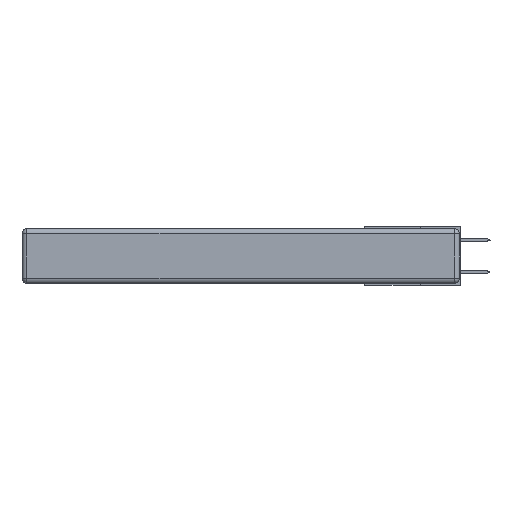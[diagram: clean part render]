
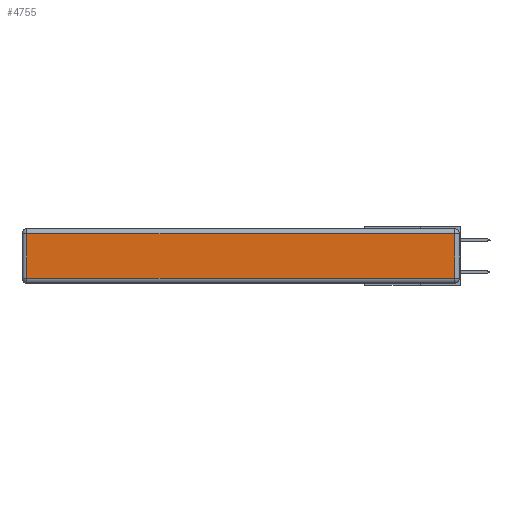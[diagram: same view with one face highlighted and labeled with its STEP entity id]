
A CAD part, left-side view. The second image highlights one B-rep face of the part: STEP entity #4755.
In plain terms, the highlighted planar face has unit normal (-1, 0, 0).
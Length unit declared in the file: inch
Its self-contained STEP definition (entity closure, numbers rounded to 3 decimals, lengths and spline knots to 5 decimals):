
#144 = VECTOR ( 'NONE', #8785, 39.37008 ) ;
#2497 = EDGE_CURVE ( 'NONE', #9733, #4159, #14385, .T. ) ;
#2549 = CARTESIAN_POINT ( 'NONE',  ( 0., 0.03, -0.313 ) ) ;
#3283 = LINE ( 'NONE', #12696, #7405 ) ;
#3413 = VECTOR ( 'NONE', #4306, 39.37008 ) ;
#3564 = DIRECTION ( 'NONE',  ( 0., 1., 0. ) ) ;
#3847 = LINE ( 'NONE', #7568, #144 ) ;
#4159 = VERTEX_POINT ( 'NONE', #8038 ) ;
#4306 = DIRECTION ( 'NONE',  ( 0., -1., 0. ) ) ;
#4515 = ORIENTED_EDGE ( 'NONE', *, *, #11429, .T. ) ;
#4755 = ADVANCED_FACE ( 'NONE', ( #17570 ), #12852, .T. ) ;
#5705 = ORIENTED_EDGE ( 'NONE', *, *, #2497, .T. ) ;
#7132 = CARTESIAN_POINT ( 'NONE',  ( 0., 2.72, -0.313 ) ) ;
#7305 = DIRECTION ( 'NONE',  ( 0., 0., 1. ) ) ;
#7405 = VECTOR ( 'NONE', #14125, 39.37008 ) ;
#7568 = CARTESIAN_POINT ( 'NONE',  ( 0., 0.03, -0.343 ) ) ;
#8028 = VECTOR ( 'NONE', #3564, 39.37008 ) ;
#8038 = CARTESIAN_POINT ( 'NONE',  ( 0., 2.72, -0.03 ) ) ;
#8306 = CARTESIAN_POINT ( 'NONE',  ( 0., 0., -0.313 ) ) ;
#8723 = CARTESIAN_POINT ( 'NONE',  ( 0., 0.03, -0.03 ) ) ;
#8785 = DIRECTION ( 'NONE',  ( 0., 0., 1. ) ) ;
#9094 = ORIENTED_EDGE ( 'NONE', *, *, #11733, .T. ) ;
#9486 = VERTEX_POINT ( 'NONE', #2549 ) ;
#9733 = VERTEX_POINT ( 'NONE', #8723 ) ;
#10212 = DIRECTION ( 'NONE',  ( -1., 0., 0. ) ) ;
#11429 = EDGE_CURVE ( 'NONE', #16785, #9486, #12106, .T. ) ;
#11733 = EDGE_CURVE ( 'NONE', #9486, #9733, #3847, .T. ) ;
#12106 = LINE ( 'NONE', #8306, #3413 ) ;
#12696 = CARTESIAN_POINT ( 'NONE',  ( 0., 2.72, -0.343 ) ) ;
#12852 = PLANE ( 'NONE',  #15052 ) ;
#14125 = DIRECTION ( 'NONE',  ( 0., 0., -1. ) ) ;
#14385 = LINE ( 'NONE', #17122, #8028 ) ;
#15052 = AXIS2_PLACEMENT_3D ( 'NONE', #15671, #10212, #7305 ) ;
#15671 = CARTESIAN_POINT ( 'NONE',  ( 0., 0., -0.343 ) ) ;
#16258 = EDGE_CURVE ( 'NONE', #4159, #16785, #3283, .T. ) ;
#16304 = ORIENTED_EDGE ( 'NONE', *, *, #16258, .T. ) ;
#16754 = EDGE_LOOP ( 'NONE', ( #4515, #9094, #5705, #16304 ) ) ;
#16785 = VERTEX_POINT ( 'NONE', #7132 ) ;
#17122 = CARTESIAN_POINT ( 'NONE',  ( 0., 2.75, -0.03 ) ) ;
#17570 = FACE_OUTER_BOUND ( 'NONE', #16754, .T. ) ;
